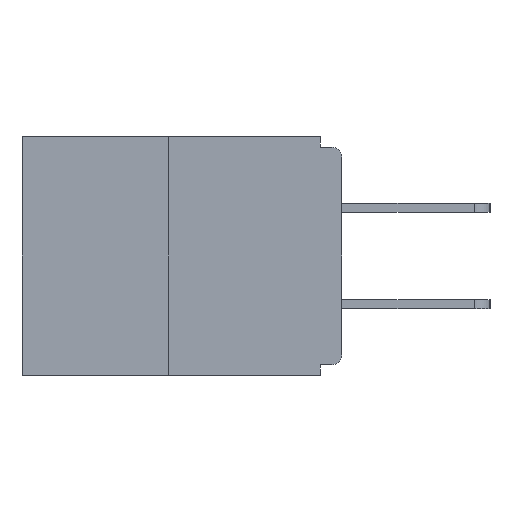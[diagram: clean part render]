
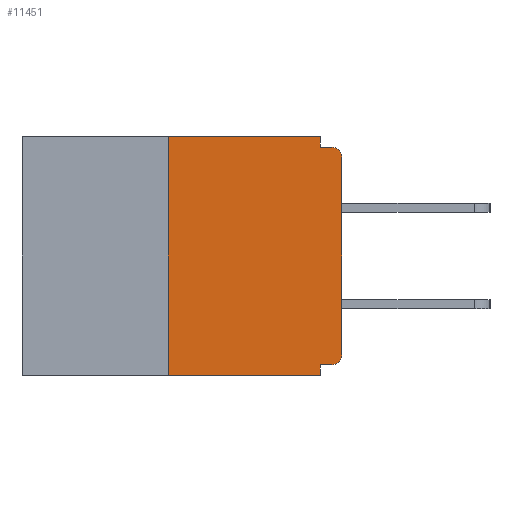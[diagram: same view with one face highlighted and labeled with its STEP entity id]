
A CAD part, left-side view. The second image highlights one B-rep face of the part: STEP entity #11451.
In plain terms, the highlighted planar face has unit normal (-1, 0, 0).
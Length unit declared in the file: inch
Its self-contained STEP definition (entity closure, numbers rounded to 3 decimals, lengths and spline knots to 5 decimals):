
#53 = VECTOR ( 'NONE', #5472, 39.37008 ) ;
#412 = ORIENTED_EDGE ( 'NONE', *, *, #5192, .F. ) ;
#585 = CARTESIAN_POINT ( 'NONE',  ( 0., 0.25, 0. ) ) ;
#654 = VERTEX_POINT ( 'NONE', #6298 ) ;
#674 = VECTOR ( 'NONE', #7623, 39.37008 ) ;
#743 = ORIENTED_EDGE ( 'NONE', *, *, #8570, .F. ) ;
#1623 = DIRECTION ( 'NONE',  ( 1., 0., 0. ) ) ;
#1670 = DIRECTION ( 'NONE',  ( 0., 0., -1. ) ) ;
#2189 = CARTESIAN_POINT ( 'NONE',  ( 0., 0.46, -0.343 ) ) ;
#2380 = CARTESIAN_POINT ( 'NONE',  ( 0., 0.031, -0.343 ) ) ;
#2381 = AXIS2_PLACEMENT_3D ( 'NONE', #4638, #1623, #1670 ) ;
#2440 = DIRECTION ( 'NONE',  ( 0., 0., 1. ) ) ;
#2556 = VERTEX_POINT ( 'NONE', #8159 ) ;
#2804 = VERTEX_POINT ( 'NONE', #7552 ) ;
#2878 = VERTEX_POINT ( 'NONE', #11427 ) ;
#3375 = LINE ( 'NONE', #4517, #674 ) ;
#3436 = ORIENTED_EDGE ( 'NONE', *, *, #8036, .T. ) ;
#3502 = DIRECTION ( 'NONE',  ( 0., 0., -1. ) ) ;
#3613 = VECTOR ( 'NONE', #3502, 39.37008 ) ;
#3891 = ORIENTED_EDGE ( 'NONE', *, *, #4797, .T. ) ;
#4048 = VECTOR ( 'NONE', #5160, 39.37008 ) ;
#4320 = AXIS2_PLACEMENT_3D ( 'NONE', #5761, #12798, #6808 ) ;
#4517 = CARTESIAN_POINT ( 'NONE',  ( 0., 0., -0.328 ) ) ;
#4638 = CARTESIAN_POINT ( 'NONE',  ( 0., 0.46, 0. ) ) ;
#4640 = ORIENTED_EDGE ( 'NONE', *, *, #12644, .F. ) ;
#4663 = CARTESIAN_POINT ( 'NONE',  ( 0., 0.25, -0.343 ) ) ;
#4730 = DIRECTION ( 'NONE',  ( -1., 0., 0. ) ) ;
#4797 = EDGE_CURVE ( 'NONE', #10413, #10653, #11500, .T. ) ;
#4867 = DIRECTION ( 'NONE',  ( 0., 0., -1. ) ) ;
#5022 = CARTESIAN_POINT ( 'NONE',  ( 0., 0.031, -0.015 ) ) ;
#5160 = DIRECTION ( 'NONE',  ( 0., -1., 0. ) ) ;
#5192 = EDGE_CURVE ( 'NONE', #9705, #6979, #5626, .T. ) ;
#5315 = CARTESIAN_POINT ( 'NONE',  ( 0., 0., 0. ) ) ;
#5472 = DIRECTION ( 'NONE',  ( 0., 0., -1. ) ) ;
#5626 = LINE ( 'NONE', #585, #6276 ) ;
#5695 = VERTEX_POINT ( 'NONE', #7757 ) ;
#5712 = VECTOR ( 'NONE', #10341, 39.37008 ) ;
#5761 = CARTESIAN_POINT ( 'NONE',  ( 0., 0.015, -0.03 ) ) ;
#5930 = LINE ( 'NONE', #2380, #53 ) ;
#6065 = CARTESIAN_POINT ( 'NONE',  ( 0., 0.46, 0. ) ) ;
#6245 = ORIENTED_EDGE ( 'NONE', *, *, #12251, .T. ) ;
#6276 = VECTOR ( 'NONE', #7772, 39.37008 ) ;
#6298 = CARTESIAN_POINT ( 'NONE',  ( 0., 0.031, 0. ) ) ;
#6451 = VERTEX_POINT ( 'NONE', #5022 ) ;
#6808 = DIRECTION ( 'NONE',  ( 0., 0., -1. ) ) ;
#6968 = CARTESIAN_POINT ( 'NONE',  ( 0., 0., -0.313 ) ) ;
#6979 = VERTEX_POINT ( 'NONE', #8870 ) ;
#7146 = ORIENTED_EDGE ( 'NONE', *, *, #11625, .F. ) ;
#7277 = ORIENTED_EDGE ( 'NONE', *, *, #7616, .T. ) ;
#7552 = CARTESIAN_POINT ( 'NONE',  ( 0., 0.031, -0.328 ) ) ;
#7616 = EDGE_CURVE ( 'NONE', #9705, #2556, #8287, .T. ) ;
#7623 = DIRECTION ( 'NONE',  ( 0., 1., 0. ) ) ;
#7733 = LINE ( 'NONE', #6065, #4048 ) ;
#7757 = CARTESIAN_POINT ( 'NONE',  ( 0., 0., -0.03 ) ) ;
#7772 = DIRECTION ( 'NONE',  ( 0., 0., 1. ) ) ;
#8036 = EDGE_CURVE ( 'NONE', #10653, #5695, #11707, .T. ) ;
#8105 = LINE ( 'NONE', #10497, #3613 ) ;
#8159 = CARTESIAN_POINT ( 'NONE',  ( 0., 0.031, -0.343 ) ) ;
#8287 = LINE ( 'NONE', #2189, #5712 ) ;
#8304 = ORIENTED_EDGE ( 'NONE', *, *, #13081, .F. ) ;
#8329 = VECTOR ( 'NONE', #12203, 39.37008 ) ;
#8528 = FACE_OUTER_BOUND ( 'NONE', #12023, .T. ) ;
#8570 = EDGE_CURVE ( 'NONE', #654, #6451, #8105, .T. ) ;
#8870 = CARTESIAN_POINT ( 'NONE',  ( 0., 0.25, 0. ) ) ;
#8889 = PLANE ( 'NONE',  #2381 ) ;
#9051 = VECTOR ( 'NONE', #2440, 39.37008 ) ;
#9403 = LINE ( 'NONE', #10908, #8329 ) ;
#9559 = ORIENTED_EDGE ( 'NONE', *, *, #12981, .F. ) ;
#9629 = AXIS2_PLACEMENT_3D ( 'NONE', #9852, #4730, #4867 ) ;
#9705 = VERTEX_POINT ( 'NONE', #4663 ) ;
#9852 = CARTESIAN_POINT ( 'NONE',  ( 0., 0.015, -0.313 ) ) ;
#10341 = DIRECTION ( 'NONE',  ( 0., -1., 0. ) ) ;
#10413 = VERTEX_POINT ( 'NONE', #10700 ) ;
#10497 = CARTESIAN_POINT ( 'NONE',  ( 0., 0.031, 0. ) ) ;
#10653 = VERTEX_POINT ( 'NONE', #6968 ) ;
#10700 = CARTESIAN_POINT ( 'NONE',  ( 0., 0.015, -0.328 ) ) ;
#10908 = CARTESIAN_POINT ( 'NONE',  ( 0., 0., -0.015 ) ) ;
#11427 = CARTESIAN_POINT ( 'NONE',  ( 0., 0.015, -0.015 ) ) ;
#11451 = ADVANCED_FACE ( 'NONE', ( #8528 ), #8889, .F. ) ;
#11500 = CIRCLE ( 'NONE', #9629, 0.015 ) ;
#11625 = EDGE_CURVE ( 'NONE', #6979, #654, #7733, .T. ) ;
#11707 = LINE ( 'NONE', #5315, #9051 ) ;
#12023 = EDGE_LOOP ( 'NONE', ( #7146, #412, #7277, #4640, #9559, #3891, #3436, #6245, #8304, #743 ) ) ;
#12203 = DIRECTION ( 'NONE',  ( 0., -1., 0. ) ) ;
#12251 = EDGE_CURVE ( 'NONE', #5695, #2878, #12393, .T. ) ;
#12393 = CIRCLE ( 'NONE', #4320, 0.015 ) ;
#12644 = EDGE_CURVE ( 'NONE', #2804, #2556, #5930, .T. ) ;
#12798 = DIRECTION ( 'NONE',  ( -1., 0., 0. ) ) ;
#12981 = EDGE_CURVE ( 'NONE', #10413, #2804, #3375, .T. ) ;
#13081 = EDGE_CURVE ( 'NONE', #6451, #2878, #9403, .T. ) ;
